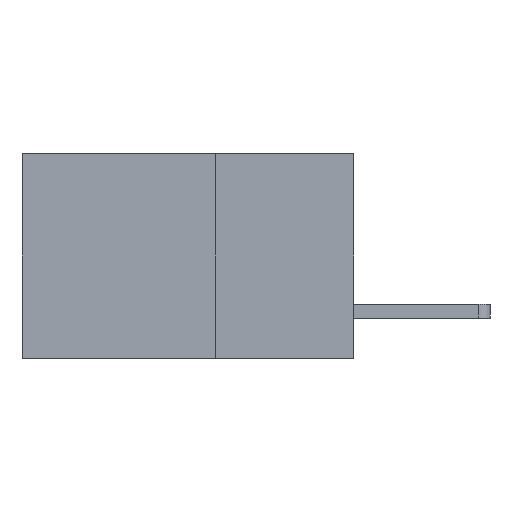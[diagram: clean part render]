
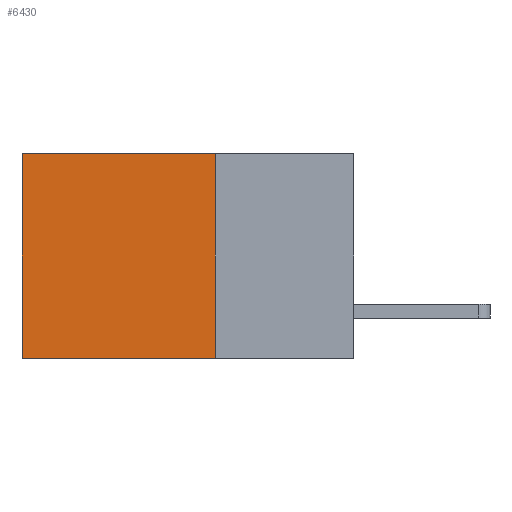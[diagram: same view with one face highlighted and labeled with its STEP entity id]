
A CAD part, left-side view. The second image highlights one B-rep face of the part: STEP entity #6430.
In plain terms, the highlighted planar face has unit normal (-1, 0, 0).
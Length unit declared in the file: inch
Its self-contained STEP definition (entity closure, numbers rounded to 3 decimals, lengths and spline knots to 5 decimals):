
#321 = VERTEX_POINT ( 'NONE', #6943 ) ;
#350 = DIRECTION ( 'NONE',  ( 0., 0., -1. ) ) ;
#459 = VERTEX_POINT ( 'NONE', #9277 ) ;
#663 = FACE_OUTER_BOUND ( 'NONE', #7089, .T. ) ;
#1570 = EDGE_CURVE ( 'NONE', #321, #8442, #5824, .T. ) ;
#1733 = DIRECTION ( 'NONE',  ( 0., 1., 0. ) ) ;
#2993 = DIRECTION ( 'NONE',  ( 0., 0., -1. ) ) ;
#3197 = AXIS2_PLACEMENT_3D ( 'NONE', #5838, #4446, #2993 ) ;
#3205 = LINE ( 'NONE', #6245, #6541 ) ;
#3354 = CARTESIAN_POINT ( 'NONE',  ( 0.2875, 0.6, 0. ) ) ;
#3682 = VECTOR ( 'NONE', #4981, 39.37008 ) ;
#4335 = CARTESIAN_POINT ( 'NONE',  ( 0.2875, 0.25, 0. ) ) ;
#4446 = DIRECTION ( 'NONE',  ( 1., 0., 0. ) ) ;
#4594 = ORIENTED_EDGE ( 'NONE', *, *, #8661, .F. ) ;
#4981 = DIRECTION ( 'NONE',  ( 0., 0., -1. ) ) ;
#5357 = CARTESIAN_POINT ( 'NONE',  ( 0.2875, 0.6, 0. ) ) ;
#5630 = CARTESIAN_POINT ( 'NONE',  ( 0.2875, 0.25, -0.37 ) ) ;
#5824 = LINE ( 'NONE', #4335, #8464 ) ;
#5838 = CARTESIAN_POINT ( 'NONE',  ( 0.2875, 0.25, 0. ) ) ;
#6106 = ORIENTED_EDGE ( 'NONE', *, *, #1570, .F. ) ;
#6245 = CARTESIAN_POINT ( 'NONE',  ( 0.2875, 0.25, 0. ) ) ;
#6332 = LINE ( 'NONE', #3354, #3682 ) ;
#6430 = ADVANCED_FACE ( 'NONE', ( #663 ), #9034, .F. ) ;
#6533 = VECTOR ( 'NONE', #9705, 39.37008 ) ;
#6541 = VECTOR ( 'NONE', #1733, 39.37008 ) ;
#6748 = EDGE_CURVE ( 'NONE', #6911, #459, #6332, .T. ) ;
#6911 = VERTEX_POINT ( 'NONE', #5357 ) ;
#6943 = CARTESIAN_POINT ( 'NONE',  ( 0.2875, 0.25, 0. ) ) ;
#7089 = EDGE_LOOP ( 'NONE', ( #8909, #4594, #6106, #7141 ) ) ;
#7141 = ORIENTED_EDGE ( 'NONE', *, *, #9140, .T. ) ;
#8066 = CARTESIAN_POINT ( 'NONE',  ( 0.2875, 0.25, -0.37 ) ) ;
#8164 = LINE ( 'NONE', #8066, #6533 ) ;
#8442 = VERTEX_POINT ( 'NONE', #5630 ) ;
#8464 = VECTOR ( 'NONE', #350, 39.37008 ) ;
#8661 = EDGE_CURVE ( 'NONE', #8442, #459, #8164, .T. ) ;
#8909 = ORIENTED_EDGE ( 'NONE', *, *, #6748, .T. ) ;
#9034 = PLANE ( 'NONE',  #3197 ) ;
#9140 = EDGE_CURVE ( 'NONE', #321, #6911, #3205, .T. ) ;
#9277 = CARTESIAN_POINT ( 'NONE',  ( 0.2875, 0.6, -0.37 ) ) ;
#9705 = DIRECTION ( 'NONE',  ( 0., 1., 0. ) ) ;
